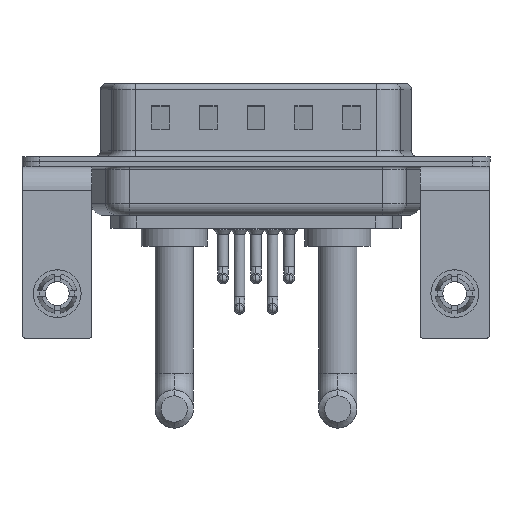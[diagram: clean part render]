
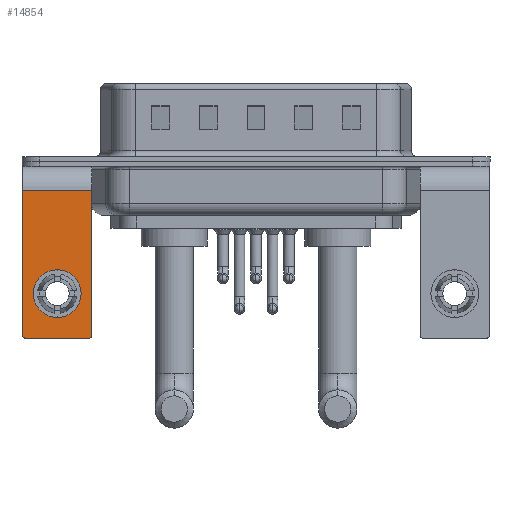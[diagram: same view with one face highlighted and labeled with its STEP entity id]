
A CAD part, front view. The second image highlights one B-rep face of the part: STEP entity #14854.
In plain terms, the highlighted planar face has unit normal (0, -1, 0).
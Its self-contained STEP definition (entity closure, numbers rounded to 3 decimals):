
#56 = VERTEX_POINT ( 'NONE', #2348 ) ;
#149 = EDGE_CURVE ( 'NONE', #22904, #11517, #3817, .T. ) ;
#185 = CARTESIAN_POINT ( 'NONE',  ( 2.9, -6.25, -14.55 ) ) ;
#507 = LINE ( 'NONE', #22277, #21273 ) ;
#567 = CARTESIAN_POINT ( 'NONE',  ( -2.9, -6.25, -2.4 ) ) ;
#894 = CARTESIAN_POINT ( 'NONE',  ( 2.9, -6.25, -2.4 ) ) ;
#913 = ORIENTED_EDGE ( 'NONE', *, *, #10003, .T. ) ;
#1874 = ORIENTED_EDGE ( 'NONE', *, *, #149, .F. ) ;
#2284 = CARTESIAN_POINT ( 'NONE',  ( 2.9, -6.25, -2.4 ) ) ;
#2348 = CARTESIAN_POINT ( 'NONE',  ( 0., -6.25, -9.07 ) ) ;
#2463 = ORIENTED_EDGE ( 'NONE', *, *, #6773, .T. ) ;
#2592 = CIRCLE ( 'NONE', #7183, 2. ) ;
#2789 = DIRECTION ( 'NONE',  ( 0., 0., 1. ) ) ;
#3043 = CARTESIAN_POINT ( 'NONE',  ( 0., -6.25, -13.07 ) ) ;
#3105 = EDGE_LOOP ( 'NONE', ( #3783, #2463 ) ) ;
#3625 = CIRCLE ( 'NONE', #11235, 0.25 ) ;
#3783 = ORIENTED_EDGE ( 'NONE', *, *, #17501, .T. ) ;
#3817 = LINE ( 'NONE', #7852, #8130 ) ;
#4199 = DIRECTION ( 'NONE',  ( 0., 0., -1. ) ) ;
#4696 = DIRECTION ( 'NONE',  ( -1., 0., 0. ) ) ;
#5200 = EDGE_CURVE ( 'NONE', #22904, #15500, #11841, .T. ) ;
#5375 = ORIENTED_EDGE ( 'NONE', *, *, #6822, .T. ) ;
#5675 = CARTESIAN_POINT ( 'NONE',  ( -2.65, -6.25, -14.55 ) ) ;
#6212 = FACE_OUTER_BOUND ( 'NONE', #20072, .T. ) ;
#6773 = EDGE_CURVE ( 'NONE', #56, #21928, #2592, .T. ) ;
#6822 = EDGE_CURVE ( 'NONE', #9949, #19641, #21605, .T. ) ;
#7067 = CARTESIAN_POINT ( 'NONE',  ( 0., -6.25, -11.07 ) ) ;
#7183 = AXIS2_PLACEMENT_3D ( 'NONE', #11022, #14352, #8884 ) ;
#7553 = AXIS2_PLACEMENT_3D ( 'NONE', #5675, #12812, #11130 ) ;
#7767 = DIRECTION ( 'NONE',  ( 0., 0., 1. ) ) ;
#7852 = CARTESIAN_POINT ( 'NONE',  ( 2.9, -6.25, -2.4 ) ) ;
#8130 = VECTOR ( 'NONE', #13417, 1000. ) ;
#8374 = ORIENTED_EDGE ( 'NONE', *, *, #16927, .T. ) ;
#8884 = DIRECTION ( 'NONE',  ( 0., 0., 1. ) ) ;
#9559 = DIRECTION ( 'NONE',  ( 0., 1., 0. ) ) ;
#9949 = VERTEX_POINT ( 'NONE', #17335 ) ;
#10003 = EDGE_CURVE ( 'NONE', #15261, #11517, #3625, .T. ) ;
#10081 = CARTESIAN_POINT ( 'NONE',  ( 2.9, -6.25, -14.8 ) ) ;
#11022 = CARTESIAN_POINT ( 'NONE',  ( 0., -6.25, -11.07 ) ) ;
#11130 = DIRECTION ( 'NONE',  ( 0., 0., 1. ) ) ;
#11235 = AXIS2_PLACEMENT_3D ( 'NONE', #16844, #19103, #2789 ) ;
#11517 = VERTEX_POINT ( 'NONE', #185 ) ;
#11841 = LINE ( 'NONE', #894, #15033 ) ;
#12465 = ORIENTED_EDGE ( 'NONE', *, *, #18139, .F. ) ;
#12812 = DIRECTION ( 'NONE',  ( 0., -1., 0. ) ) ;
#13417 = DIRECTION ( 'NONE',  ( 0., 0., -1. ) ) ;
#13649 = DIRECTION ( 'NONE',  ( -1., 0., 0. ) ) ;
#13837 = VECTOR ( 'NONE', #13649, 1000. ) ;
#14093 = CIRCLE ( 'NONE', #14851, 2. ) ;
#14352 = DIRECTION ( 'NONE',  ( 0., 1., 0. ) ) ;
#14851 = AXIS2_PLACEMENT_3D ( 'NONE', #7067, #19315, #15722 ) ;
#14854 = ADVANCED_FACE ( 'NONE', ( #20728, #6212 ), #18944, .F. ) ;
#15033 = VECTOR ( 'NONE', #4696, 1000. ) ;
#15261 = VERTEX_POINT ( 'NONE', #20471 ) ;
#15500 = VERTEX_POINT ( 'NONE', #567 ) ;
#15722 = DIRECTION ( 'NONE',  ( 0., 0., 1. ) ) ;
#15796 = CARTESIAN_POINT ( 'NONE',  ( -2.65, -6.25, -14.8 ) ) ;
#16844 = CARTESIAN_POINT ( 'NONE',  ( 2.65, -6.25, -14.55 ) ) ;
#16927 = EDGE_CURVE ( 'NONE', #15500, #9949, #507, .T. ) ;
#17335 = CARTESIAN_POINT ( 'NONE',  ( -2.9, -6.25, -14.55 ) ) ;
#17501 = EDGE_CURVE ( 'NONE', #21928, #56, #14093, .T. ) ;
#18139 = EDGE_CURVE ( 'NONE', #15261, #19641, #19342, .T. ) ;
#18944 = PLANE ( 'NONE',  #22780 ) ;
#19103 = DIRECTION ( 'NONE',  ( 0., -1., 0. ) ) ;
#19315 = DIRECTION ( 'NONE',  ( 0., 1., 0. ) ) ;
#19342 = LINE ( 'NONE', #10081, #13837 ) ;
#19641 = VERTEX_POINT ( 'NONE', #15796 ) ;
#19751 = CARTESIAN_POINT ( 'NONE',  ( 2.9, -6.25, -2.4 ) ) ;
#20072 = EDGE_LOOP ( 'NONE', ( #8374, #5375, #12465, #913, #1874, #21481 ) ) ;
#20471 = CARTESIAN_POINT ( 'NONE',  ( 2.65, -6.25, -14.8 ) ) ;
#20728 = FACE_BOUND ( 'NONE', #3105, .T. ) ;
#21273 = VECTOR ( 'NONE', #4199, 1000. ) ;
#21481 = ORIENTED_EDGE ( 'NONE', *, *, #5200, .T. ) ;
#21605 = CIRCLE ( 'NONE', #7553, 0.25 ) ;
#21928 = VERTEX_POINT ( 'NONE', #3043 ) ;
#22277 = CARTESIAN_POINT ( 'NONE',  ( -2.9, -6.25, -2.4 ) ) ;
#22780 = AXIS2_PLACEMENT_3D ( 'NONE', #2284, #9559, #7767 ) ;
#22904 = VERTEX_POINT ( 'NONE', #19751 ) ;
